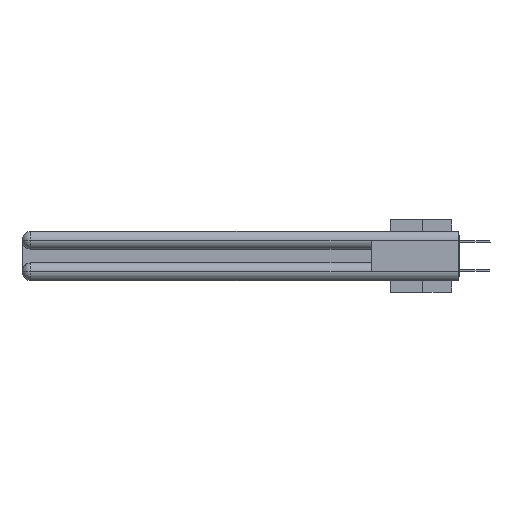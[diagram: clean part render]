
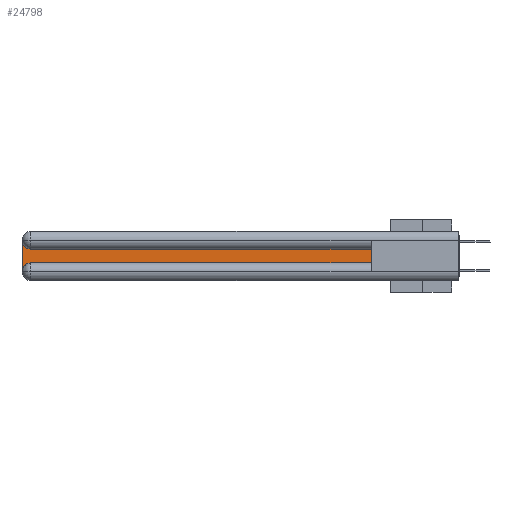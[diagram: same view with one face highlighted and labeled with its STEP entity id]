
A CAD part, left-side view. The second image highlights one B-rep face of the part: STEP entity #24798.
In plain terms, the highlighted planar face has unit normal (-1, 0, 0).
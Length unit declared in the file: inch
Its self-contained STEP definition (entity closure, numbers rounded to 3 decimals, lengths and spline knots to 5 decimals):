
#175 = ORIENTED_EDGE ( 'NONE', *, *, #2531, .T. ) ;
#392 = CARTESIAN_POINT ( 'NONE',  ( 0.075, 2.94, -0.2175 ) ) ;
#464 = DIRECTION ( 'NONE',  ( 1., 0., 0. ) ) ;
#1629 = DIRECTION ( 'NONE',  ( 1., 0., 0. ) ) ;
#2531 = EDGE_CURVE ( 'NONE', #21586, #13815, #28326, .T. ) ;
#3858 = ORIENTED_EDGE ( 'NONE', *, *, #19100, .T. ) ;
#4198 = EDGE_CURVE ( 'NONE', #28854, #12945, #4352, .T. ) ;
#4352 = LINE ( 'NONE', #10340, #15996 ) ;
#8010 = EDGE_CURVE ( 'NONE', #20808, #21586, #14670, .T. ) ;
#8018 = CARTESIAN_POINT ( 'NONE',  ( 0.075, 0.6, -0.1225 ) ) ;
#8721 = AXIS2_PLACEMENT_3D ( 'NONE', #15510, #1629, #17944 ) ;
#8731 = CARTESIAN_POINT ( 'NONE',  ( 0.075, 3., -0.1225 ) ) ;
#9614 = EDGE_CURVE ( 'NONE', #12945, #20808, #16785, .T. ) ;
#9781 = DIRECTION ( 'NONE',  ( 0., 1., 0. ) ) ;
#10048 = CARTESIAN_POINT ( 'NONE',  ( 0.075, 3., -0.2775 ) ) ;
#10340 = CARTESIAN_POINT ( 'NONE',  ( 0.075, 0.6, -0.2175 ) ) ;
#11394 = AXIS2_PLACEMENT_3D ( 'NONE', #19305, #464, #21450 ) ;
#11712 = VECTOR ( 'NONE', #15534, 39.37008 ) ;
#12008 = CARTESIAN_POINT ( 'NONE',  ( 0.075, 0.6, -0.1225 ) ) ;
#12319 = VECTOR ( 'NONE', #29527, 39.37008 ) ;
#12681 = LINE ( 'NONE', #24883, #12319 ) ;
#12945 = VERTEX_POINT ( 'NONE', #22850 ) ;
#13139 = CARTESIAN_POINT ( 'NONE',  ( 0.075, 2.94, -0.1225 ) ) ;
#13815 = VERTEX_POINT ( 'NONE', #23597 ) ;
#14126 = VERTEX_POINT ( 'NONE', #10048 ) ;
#14404 = AXIS2_PLACEMENT_3D ( 'NONE', #8731, #15232, #15328 ) ;
#14670 = LINE ( 'NONE', #12008, #28801 ) ;
#15232 = DIRECTION ( 'NONE',  ( 1., 0., 0. ) ) ;
#15328 = DIRECTION ( 'NONE',  ( 0., 0., -1. ) ) ;
#15359 = FACE_OUTER_BOUND ( 'NONE', #18610, .T. ) ;
#15510 = CARTESIAN_POINT ( 'NONE',  ( 0.075, 2.94, -0.2775 ) ) ;
#15534 = DIRECTION ( 'NONE',  ( 0., 0., 1. ) ) ;
#15636 = CARTESIAN_POINT ( 'NONE',  ( 0.075, 0.6, -0.2175 ) ) ;
#15996 = VECTOR ( 'NONE', #17557, 39.37008 ) ;
#16525 = ORIENTED_EDGE ( 'NONE', *, *, #9614, .T. ) ;
#16785 = LINE ( 'NONE', #15636, #11712 ) ;
#17557 = DIRECTION ( 'NONE',  ( 0., -1., 0. ) ) ;
#17944 = DIRECTION ( 'NONE',  ( 0., 0., -1. ) ) ;
#18610 = EDGE_LOOP ( 'NONE', ( #25162, #175, #3858, #28700, #24229, #16525 ) ) ;
#19100 = EDGE_CURVE ( 'NONE', #13815, #14126, #12681, .T. ) ;
#19305 = CARTESIAN_POINT ( 'NONE',  ( 0.075, 2.94, -0.0625 ) ) ;
#19744 = EDGE_CURVE ( 'NONE', #14126, #28854, #22097, .T. ) ;
#19982 = PLANE ( 'NONE',  #14404 ) ;
#20808 = VERTEX_POINT ( 'NONE', #8018 ) ;
#21450 = DIRECTION ( 'NONE',  ( 0., 0., -1. ) ) ;
#21586 = VERTEX_POINT ( 'NONE', #13139 ) ;
#22097 = CIRCLE ( 'NONE', #8721, 0.06 ) ;
#22850 = CARTESIAN_POINT ( 'NONE',  ( 0.075, 0.6, -0.2175 ) ) ;
#23597 = CARTESIAN_POINT ( 'NONE',  ( 0.075, 3., -0.0625 ) ) ;
#24229 = ORIENTED_EDGE ( 'NONE', *, *, #4198, .T. ) ;
#24798 = ADVANCED_FACE ( 'NONE', ( #15359 ), #19982, .F. ) ;
#24883 = CARTESIAN_POINT ( 'NONE',  ( 0.075, 3., -0.2175 ) ) ;
#25162 = ORIENTED_EDGE ( 'NONE', *, *, #8010, .T. ) ;
#28326 = CIRCLE ( 'NONE', #11394, 0.06 ) ;
#28700 = ORIENTED_EDGE ( 'NONE', *, *, #19744, .T. ) ;
#28801 = VECTOR ( 'NONE', #9781, 39.37008 ) ;
#28854 = VERTEX_POINT ( 'NONE', #392 ) ;
#29527 = DIRECTION ( 'NONE',  ( 0., 0., -1. ) ) ;
